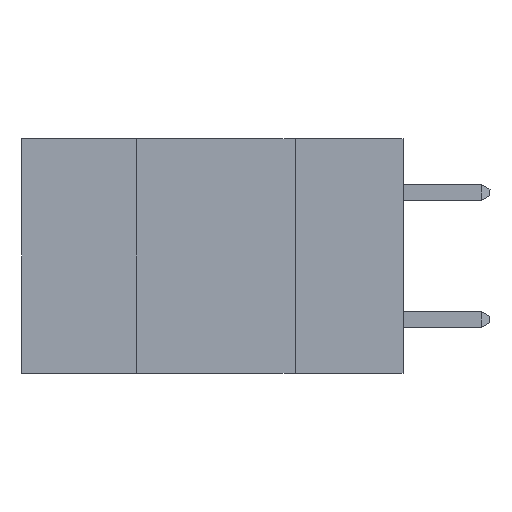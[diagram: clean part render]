
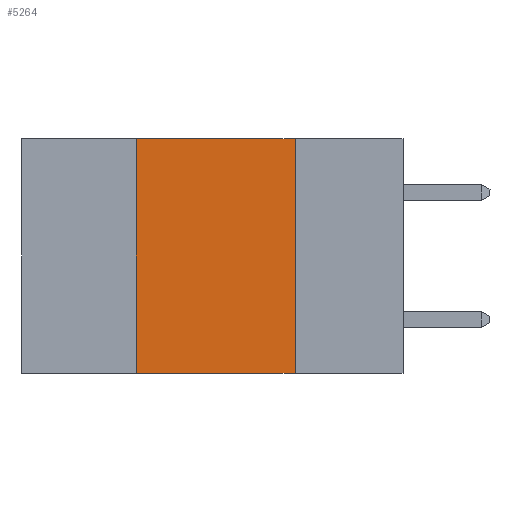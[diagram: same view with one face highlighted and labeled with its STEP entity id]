
A CAD part, left-side view. The second image highlights one B-rep face of the part: STEP entity #5264.
In plain terms, the highlighted planar face has unit normal (-1, 0, 0).
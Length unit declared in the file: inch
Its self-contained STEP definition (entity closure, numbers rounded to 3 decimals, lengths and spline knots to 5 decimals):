
#740 = LINE ( 'NONE', #7071, #5597 ) ;
#1178 = DIRECTION ( 'NONE',  ( 0., 0., 1. ) ) ;
#1287 = EDGE_CURVE ( 'NONE', #7193, #1369, #740, .T. ) ;
#1369 = VERTEX_POINT ( 'NONE', #2112 ) ;
#1387 = DIRECTION ( 'NONE',  ( 0., -1., 0. ) ) ;
#1461 = LINE ( 'NONE', #6954, #11452 ) ;
#2112 = CARTESIAN_POINT ( 'NONE',  ( 0., 0.17, 0. ) ) ;
#2247 = LINE ( 'NONE', #5561, #7061 ) ;
#3807 = PLANE ( 'NONE',  #4021 ) ;
#3824 = ORIENTED_EDGE ( 'NONE', *, *, #9845, .T. ) ;
#4021 = AXIS2_PLACEMENT_3D ( 'NONE', #5733, #10404, #4805 ) ;
#4741 = DIRECTION ( 'NONE',  ( 0., -1., 0. ) ) ;
#4805 = DIRECTION ( 'NONE',  ( 0., 0., -1. ) ) ;
#5264 = ADVANCED_FACE ( 'NONE', ( #8353 ), #3807, .F. ) ;
#5473 = EDGE_CURVE ( 'NONE', #5506, #7193, #1461, .T. ) ;
#5506 = VERTEX_POINT ( 'NONE', #6070 ) ;
#5561 = CARTESIAN_POINT ( 'NONE',  ( 0., 0.17, 0. ) ) ;
#5597 = VECTOR ( 'NONE', #4741, 39.37008 ) ;
#5733 = CARTESIAN_POINT ( 'NONE',  ( 0., 0.6, 0. ) ) ;
#6040 = ORIENTED_EDGE ( 'NONE', *, *, #5473, .F. ) ;
#6070 = CARTESIAN_POINT ( 'NONE',  ( 0., 0.42, -0.37 ) ) ;
#6151 = CARTESIAN_POINT ( 'NONE',  ( 0., 0.17, -0.37 ) ) ;
#6557 = DIRECTION ( 'NONE',  ( 0., 0., -1. ) ) ;
#6954 = CARTESIAN_POINT ( 'NONE',  ( 0., 0.42, 0. ) ) ;
#7061 = VECTOR ( 'NONE', #6557, 39.37008 ) ;
#7071 = CARTESIAN_POINT ( 'NONE',  ( 0., 0.6, 0. ) ) ;
#7153 = CARTESIAN_POINT ( 'NONE',  ( 0., 0.6, -0.37 ) ) ;
#7193 = VERTEX_POINT ( 'NONE', #8478 ) ;
#7804 = VECTOR ( 'NONE', #1387, 39.37008 ) ;
#8353 = FACE_OUTER_BOUND ( 'NONE', #10207, .T. ) ;
#8478 = CARTESIAN_POINT ( 'NONE',  ( 0., 0.42, 0. ) ) ;
#9095 = VERTEX_POINT ( 'NONE', #6151 ) ;
#9355 = ORIENTED_EDGE ( 'NONE', *, *, #11206, .F. ) ;
#9845 = EDGE_CURVE ( 'NONE', #5506, #9095, #10284, .T. ) ;
#10207 = EDGE_LOOP ( 'NONE', ( #9355, #10302, #6040, #3824 ) ) ;
#10284 = LINE ( 'NONE', #7153, #7804 ) ;
#10302 = ORIENTED_EDGE ( 'NONE', *, *, #1287, .F. ) ;
#10404 = DIRECTION ( 'NONE',  ( 1., 0., 0. ) ) ;
#11206 = EDGE_CURVE ( 'NONE', #1369, #9095, #2247, .T. ) ;
#11452 = VECTOR ( 'NONE', #1178, 39.37008 ) ;
